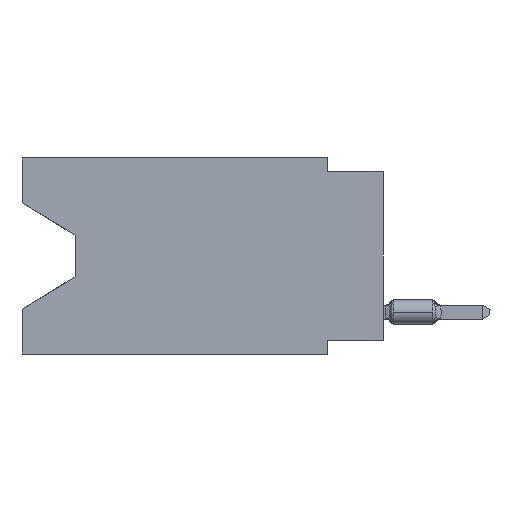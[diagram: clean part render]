
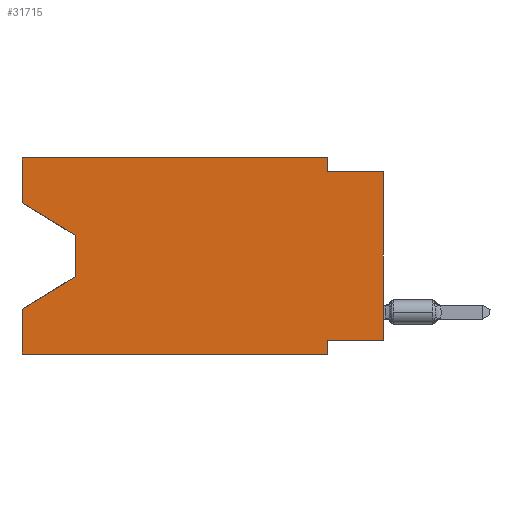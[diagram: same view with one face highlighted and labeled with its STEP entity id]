
A CAD part, left-side view. The second image highlights one B-rep face of the part: STEP entity #31715.
In plain terms, the highlighted planar face has unit normal (-1, 0, 0).
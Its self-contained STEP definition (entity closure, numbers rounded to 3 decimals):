
#125 = CARTESIAN_POINT ( 'NONE',  ( 0., 0., -8.255 ) ) ;
#251 = VECTOR ( 'NONE', #24260, 1000. ) ;
#558 = VERTEX_POINT ( 'NONE', #2072 ) ;
#775 = EDGE_CURVE ( 'NONE', #17953, #24362, #17865, .T. ) ;
#1109 = EDGE_CURVE ( 'NONE', #20200, #25573, #2750, .T. ) ;
#1772 = CARTESIAN_POINT ( 'NONE',  ( 0., 16.383, -8.89 ) ) ;
#1824 = LINE ( 'NONE', #4504, #5482 ) ;
#2072 = CARTESIAN_POINT ( 'NONE',  ( 0., 13.97, -5.385 ) ) ;
#2085 = VERTEX_POINT ( 'NONE', #31801 ) ;
#2093 = LINE ( 'NONE', #10641, #32458 ) ;
#2297 = CARTESIAN_POINT ( 'NONE',  ( 0., 0., -8.255 ) ) ;
#2750 = LINE ( 'NONE', #13405, #251 ) ;
#2840 = EDGE_CURVE ( 'NONE', #20200, #8524, #20620, .T. ) ;
#3469 = CARTESIAN_POINT ( 'NONE',  ( 0., 0., -0.635 ) ) ;
#3685 = CARTESIAN_POINT ( 'NONE',  ( 0., 2.54, -0.635 ) ) ;
#3745 = VECTOR ( 'NONE', #34811, 1000. ) ;
#3933 = EDGE_CURVE ( 'NONE', #8524, #24362, #25731, .T. ) ;
#4023 = CARTESIAN_POINT ( 'NONE',  ( 0., 2.54, 0. ) ) ;
#4471 = ORIENTED_EDGE ( 'NONE', *, *, #775, .T. ) ;
#4504 = CARTESIAN_POINT ( 'NONE',  ( 0., 16.383, 0. ) ) ;
#4575 = DIRECTION ( 'NONE',  ( 0., 0., -1. ) ) ;
#5482 = VECTOR ( 'NONE', #28838, 1000. ) ;
#5886 = EDGE_CURVE ( 'NONE', #2085, #13032, #15966, .T. ) ;
#6331 = EDGE_CURVE ( 'NONE', #18732, #33724, #34750, .T. ) ;
#6432 = ORIENTED_EDGE ( 'NONE', *, *, #27539, .T. ) ;
#7238 = LINE ( 'NONE', #25900, #14501 ) ;
#7644 = ORIENTED_EDGE ( 'NONE', *, *, #5886, .T. ) ;
#8283 = EDGE_CURVE ( 'NONE', #33724, #25573, #17318, .T. ) ;
#8332 = VECTOR ( 'NONE', #4575, 1000. ) ;
#8446 = EDGE_CURVE ( 'NONE', #17953, #18653, #26367, .T. ) ;
#8524 = VERTEX_POINT ( 'NONE', #24412 ) ;
#8652 = VERTEX_POINT ( 'NONE', #17277 ) ;
#8841 = VECTOR ( 'NONE', #25343, 1000. ) ;
#9092 = CARTESIAN_POINT ( 'NONE',  ( 0., 13.97, -5.385 ) ) ;
#10157 = EDGE_CURVE ( 'NONE', #13032, #558, #2093, .T. ) ;
#10420 = CARTESIAN_POINT ( 'NONE',  ( 0., 2.54, 0. ) ) ;
#10641 = CARTESIAN_POINT ( 'NONE',  ( 0., 13.97, -3.505 ) ) ;
#10683 = ORIENTED_EDGE ( 'NONE', *, *, #3933, .F. ) ;
#10754 = ORIENTED_EDGE ( 'NONE', *, *, #8283, .F. ) ;
#11823 = DIRECTION ( 'NONE',  ( 0., -1., 0. ) ) ;
#12348 = ORIENTED_EDGE ( 'NONE', *, *, #2840, .F. ) ;
#12466 = VECTOR ( 'NONE', #18023, 1000. ) ;
#12473 = ORIENTED_EDGE ( 'NONE', *, *, #27221, .F. ) ;
#12845 = CARTESIAN_POINT ( 'NONE',  ( 0., 13.97, -3.505 ) ) ;
#13032 = VERTEX_POINT ( 'NONE', #12845 ) ;
#13289 = DIRECTION ( 'NONE',  ( 0., -0.855, -0.519 ) ) ;
#13397 = AXIS2_PLACEMENT_3D ( 'NONE', #32166, #26487, #18311 ) ;
#13405 = CARTESIAN_POINT ( 'NONE',  ( 0., 0., 0. ) ) ;
#13564 = ORIENTED_EDGE ( 'NONE', *, *, #24990, .F. ) ;
#14156 = VECTOR ( 'NONE', #11823, 1000. ) ;
#14501 = VECTOR ( 'NONE', #18243, 1000. ) ;
#15304 = EDGE_LOOP ( 'NONE', ( #7644, #26237, #6432, #16644, #4471, #10683, #12348, #30804, #10754, #22174, #12473, #13564 ) ) ;
#15966 = LINE ( 'NONE', #26811, #20365 ) ;
#16377 = CARTESIAN_POINT ( 'NONE',  ( 0., 0., -0.635 ) ) ;
#16644 = ORIENTED_EDGE ( 'NONE', *, *, #8446, .F. ) ;
#17277 = CARTESIAN_POINT ( 'NONE',  ( 0., 16.383, 0. ) ) ;
#17318 = LINE ( 'NONE', #3469, #14156 ) ;
#17540 = VECTOR ( 'NONE', #29068, 1000. ) ;
#17609 = DIRECTION ( 'NONE',  ( 0., 0.855, -0.519 ) ) ;
#17621 = FACE_OUTER_BOUND ( 'NONE', #15304, .T. ) ;
#17841 = CARTESIAN_POINT ( 'NONE',  ( 0., 16.383, 0. ) ) ;
#17865 = LINE ( 'NONE', #25528, #8841 ) ;
#17953 = VERTEX_POINT ( 'NONE', #1772 ) ;
#18023 = DIRECTION ( 'NONE',  ( 0., 0., 1. ) ) ;
#18243 = DIRECTION ( 'NONE',  ( 0., 0., 1. ) ) ;
#18311 = DIRECTION ( 'NONE',  ( 0., 0., -1. ) ) ;
#18447 = DIRECTION ( 'NONE',  ( 0., 0., -1. ) ) ;
#18653 = VERTEX_POINT ( 'NONE', #21965 ) ;
#18732 = VERTEX_POINT ( 'NONE', #4023 ) ;
#20200 = VERTEX_POINT ( 'NONE', #125 ) ;
#20365 = VECTOR ( 'NONE', #13289, 1000. ) ;
#20620 = LINE ( 'NONE', #2297, #3745 ) ;
#21093 = CARTESIAN_POINT ( 'NONE',  ( 0., 2.54, -8.89 ) ) ;
#21919 = VECTOR ( 'NONE', #17609, 1000. ) ;
#21965 = CARTESIAN_POINT ( 'NONE',  ( 0., 16.383, -6.852 ) ) ;
#22174 = ORIENTED_EDGE ( 'NONE', *, *, #6331, .F. ) ;
#24260 = DIRECTION ( 'NONE',  ( 0., 0., 1. ) ) ;
#24362 = VERTEX_POINT ( 'NONE', #29868 ) ;
#24412 = CARTESIAN_POINT ( 'NONE',  ( 0., 2.54, -8.255 ) ) ;
#24990 = EDGE_CURVE ( 'NONE', #2085, #8652, #7238, .T. ) ;
#25343 = DIRECTION ( 'NONE',  ( 0., -1., 0. ) ) ;
#25528 = CARTESIAN_POINT ( 'NONE',  ( 0., 16.383, -8.89 ) ) ;
#25573 = VERTEX_POINT ( 'NONE', #16377 ) ;
#25731 = LINE ( 'NONE', #21093, #8332 ) ;
#25900 = CARTESIAN_POINT ( 'NONE',  ( 0., 16.383, 0. ) ) ;
#26237 = ORIENTED_EDGE ( 'NONE', *, *, #10157, .T. ) ;
#26367 = LINE ( 'NONE', #17841, #12466 ) ;
#26487 = DIRECTION ( 'NONE',  ( 1., 0., 0. ) ) ;
#26811 = CARTESIAN_POINT ( 'NONE',  ( 0., 16.383, -2.038 ) ) ;
#27221 = EDGE_CURVE ( 'NONE', #8652, #18732, #1824, .T. ) ;
#27539 = EDGE_CURVE ( 'NONE', #558, #18653, #33433, .T. ) ;
#28463 = PLANE ( 'NONE',  #13397 ) ;
#28838 = DIRECTION ( 'NONE',  ( 0., -1., 0. ) ) ;
#29068 = DIRECTION ( 'NONE',  ( 0., 0., -1. ) ) ;
#29868 = CARTESIAN_POINT ( 'NONE',  ( 0., 2.54, -8.89 ) ) ;
#30804 = ORIENTED_EDGE ( 'NONE', *, *, #1109, .T. ) ;
#31715 = ADVANCED_FACE ( 'NONE', ( #17621 ), #28463, .F. ) ;
#31801 = CARTESIAN_POINT ( 'NONE',  ( 0., 16.383, -2.038 ) ) ;
#32166 = CARTESIAN_POINT ( 'NONE',  ( 0., 16.383, 0. ) ) ;
#32458 = VECTOR ( 'NONE', #18447, 1000. ) ;
#33433 = LINE ( 'NONE', #9092, #21919 ) ;
#33724 = VERTEX_POINT ( 'NONE', #3685 ) ;
#34750 = LINE ( 'NONE', #10420, #17540 ) ;
#34811 = DIRECTION ( 'NONE',  ( 0., 1., 0. ) ) ;
